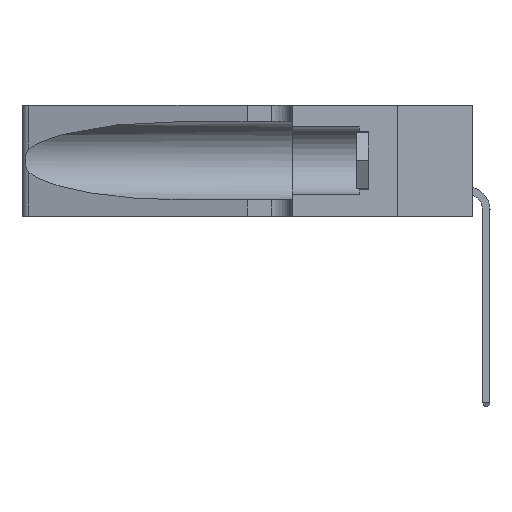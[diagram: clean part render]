
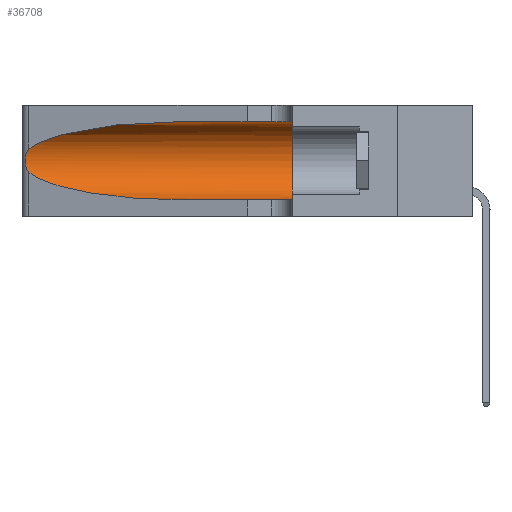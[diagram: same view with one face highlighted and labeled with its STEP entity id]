
A CAD part, left-side view. The second image highlights one B-rep face of the part: STEP entity #36708.
In plain terms, the highlighted cylindrical face has radius 3.308 mm (diameter 6.617 mm), a partial arc.
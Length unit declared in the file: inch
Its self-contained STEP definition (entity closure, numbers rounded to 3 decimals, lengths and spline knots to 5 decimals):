
#712 = CARTESIAN_POINT ( 'NONE',  ( 0.1305, 0.35, 0.185 ) ) ;
#1859 = AXIS2_PLACEMENT_3D ( 'NONE', #20855, #46440, #28651 ) ;
#2155 = EDGE_CURVE ( 'NONE', #11063, #16759, #9258, .T. ) ;
#3030 = DIRECTION ( 'NONE',  ( 0., -1., 0. ) ) ;
#3733 = ORIENTED_EDGE ( 'NONE', *, *, #29926, .T. ) ;
#4401 = CARTESIAN_POINT ( 'NONE',  ( 0.1305, 0.72297, 0.05475 ) ) ;
#5048 = CARTESIAN_POINT ( 'NONE',  ( 0.1305, 0.72297, 0.31525 ) ) ;
#6110 = EDGE_CURVE ( 'NONE', #7838, #38302, #18617, .T. ) ;
#6890 = CARTESIAN_POINT ( 'NONE',  ( 0.25487, 1.22718, 0.14631 ) ) ;
#7838 = VERTEX_POINT ( 'NONE', #35083 ) ;
#9044 = CARTESIAN_POINT ( 'NONE',  ( 0.2373, 1.15595, 0.28018 ) ) ;
#9096 = CARTESIAN_POINT ( 'NONE',  ( 0.25639, 1.23184, 0.21858 ) ) ;
#9258 =( BOUNDED_CURVE ( )  B_SPLINE_CURVE ( 3, ( #15347, #33433, #19290, #4401 ),
 .UNSPECIFIED., .F., .T. ) 
 B_SPLINE_CURVE_WITH_KNOTS ( ( 4, 4 ),
 ( 3.44316, 4.71239 ),
 .UNSPECIFIED. ) 
 CURVE ( )  GEOMETRIC_REPRESENTATION_ITEM ( )  RATIONAL_B_SPLINE_CURVE ( ( 1., 0.87, 0.87, 1. ) ) 
 REPRESENTATION_ITEM ( '' )  );
#9522 = ORIENTED_EDGE ( 'NONE', *, *, #32097, .F. ) ;
#10184 = ORIENTED_EDGE ( 'NONE', *, *, #16195, .T. ) ;
#11063 = VERTEX_POINT ( 'NONE', #45719 ) ;
#11932 = ORIENTED_EDGE ( 'NONE', *, *, #17534, .T. ) ;
#12338 = CARTESIAN_POINT ( 'NONE',  ( 0.25487, 1.22718, 0.22369 ) ) ;
#12715 = CARTESIAN_POINT ( 'NONE',  ( 0.25787, 1.23484, 0.2124 ) ) ;
#15347 = CARTESIAN_POINT ( 'NONE',  ( 0.25487, 1.22718, 0.14631 ) ) ;
#16195 = EDGE_CURVE ( 'NONE', #16759, #22867, #17653, .T. ) ;
#16316 = CARTESIAN_POINT ( 'NONE',  ( 0.1305, 0.35, 0.31525 ) ) ;
#16713 = CARTESIAN_POINT ( 'NONE',  ( 0.26017, 1.23833, 0.17102 ) ) ;
#16759 = VERTEX_POINT ( 'NONE', #20033 ) ;
#16831 = B_SPLINE_CURVE_WITH_KNOTS ( 'NONE', 3,
 ( #30952, #24330, #9096, #12715, #38059, #41662, #34634, #41838, #16713, #42008, #20325, #23975, #42804, #6890 ),
 .UNSPECIFIED., .F., .F.,
 ( 4, 2, 2, 2, 2, 2, 4 ),
 ( 0., 0.00027, 0.00053, 0.00107, 0.0016, 0.00187, 0.00214 ),
 .UNSPECIFIED. ) ;
#17534 = EDGE_CURVE ( 'NONE', #7838, #41190, #37066, .T. ) ;
#17653 = LINE ( 'NONE', #33801, #40776 ) ;
#18617 = LINE ( 'NONE', #31819, #38499 ) ;
#19290 = CARTESIAN_POINT ( 'NONE',  ( 0.18966, 0.96281, 0.05475 ) ) ;
#20033 = CARTESIAN_POINT ( 'NONE',  ( 0.1305, 0.72297, 0.05475 ) ) ;
#20325 = CARTESIAN_POINT ( 'NONE',  ( 0.25789, 1.23486, 0.15765 ) ) ;
#20855 = CARTESIAN_POINT ( 'NONE',  ( 0.1305, 1.61858, 0.185 ) ) ;
#22108 = CARTESIAN_POINT ( 'NONE',  ( 0.25487, 1.22718, 0.22369 ) ) ;
#22867 = VERTEX_POINT ( 'NONE', #43048 ) ;
#23152 = DIRECTION ( 'NONE',  ( 0., -1., 0. ) ) ;
#23975 = CARTESIAN_POINT ( 'NONE',  ( 0.25639, 1.23186, 0.15144 ) ) ;
#24330 = CARTESIAN_POINT ( 'NONE',  ( 0.25555, 1.22994, 0.2215 ) ) ;
#26096 = DIRECTION ( 'NONE',  ( 0., 0., 1. ) ) ;
#26104 = FACE_OUTER_BOUND ( 'NONE', #38270, .T. ) ;
#26655 = ORIENTED_EDGE ( 'NONE', *, *, #2155, .T. ) ;
#26684 = CYLINDRICAL_SURFACE ( 'NONE', #1859, 0.13025 ) ;
#27728 = CIRCLE ( 'NONE', #39976, 0.13025 ) ;
#28651 = DIRECTION ( 'NONE',  ( 0., 0., -1. ) ) ;
#29926 = EDGE_CURVE ( 'NONE', #41190, #11063, #16831, .T. ) ;
#30432 = ORIENTED_EDGE ( 'NONE', *, *, #6110, .F. ) ;
#30952 = CARTESIAN_POINT ( 'NONE',  ( 0.25487, 1.22718, 0.22369 ) ) ;
#31819 = CARTESIAN_POINT ( 'NONE',  ( 0.1305, 1.61858, 0.31525 ) ) ;
#32097 = EDGE_CURVE ( 'NONE', #38302, #22867, #27728, .T. ) ;
#33433 = CARTESIAN_POINT ( 'NONE',  ( 0.2373, 1.15595, 0.08982 ) ) ;
#33801 = CARTESIAN_POINT ( 'NONE',  ( 0.1305, 1.61858, 0.05475 ) ) ;
#34634 = CARTESIAN_POINT ( 'NONE',  ( 0.26075, 1.23896, 0.19203 ) ) ;
#35083 = CARTESIAN_POINT ( 'NONE',  ( 0.1305, 0.72297, 0.31525 ) ) ;
#36708 = ADVANCED_FACE ( 'NONE', ( #26104 ), #26684, .F. ) ;
#37066 =( BOUNDED_CURVE ( )  B_SPLINE_CURVE ( 3, ( #5048, #37850, #9044, #12338 ),
 .UNSPECIFIED., .F., .F. ) 
 B_SPLINE_CURVE_WITH_KNOTS ( ( 4, 4 ),
 ( 1.5708, 2.84003 ),
 .UNSPECIFIED. ) 
 CURVE ( )  GEOMETRIC_REPRESENTATION_ITEM ( )  RATIONAL_B_SPLINE_CURVE ( ( 1., 0.87, 0.87, 1. ) ) 
 REPRESENTATION_ITEM ( '' )  );
#37850 = CARTESIAN_POINT ( 'NONE',  ( 0.18966, 0.96281, 0.31525 ) ) ;
#38059 = CARTESIAN_POINT ( 'NONE',  ( 0.25854, 1.2359, 0.20912 ) ) ;
#38270 = EDGE_LOOP ( 'NONE', ( #11932, #3733, #26655, #10184, #9522, #30432 ) ) ;
#38302 = VERTEX_POINT ( 'NONE', #16316 ) ;
#38499 = VECTOR ( 'NONE', #3030, 39.37008 ) ;
#39976 = AXIS2_PLACEMENT_3D ( 'NONE', #712, #40508, #26096 ) ;
#40508 = DIRECTION ( 'NONE',  ( 0., 1., 0. ) ) ;
#40776 = VECTOR ( 'NONE', #23152, 39.37008 ) ;
#41190 = VERTEX_POINT ( 'NONE', #22108 ) ;
#41662 = CARTESIAN_POINT ( 'NONE',  ( 0.26018, 1.23835, 0.19895 ) ) ;
#41838 = CARTESIAN_POINT ( 'NONE',  ( 0.26075, 1.23896, 0.178 ) ) ;
#42008 = CARTESIAN_POINT ( 'NONE',  ( 0.25856, 1.23593, 0.16098 ) ) ;
#42804 = CARTESIAN_POINT ( 'NONE',  ( 0.25555, 1.22993, 0.14849 ) ) ;
#43048 = CARTESIAN_POINT ( 'NONE',  ( 0.1305, 0.35, 0.05475 ) ) ;
#45719 = CARTESIAN_POINT ( 'NONE',  ( 0.25487, 1.22718, 0.14631 ) ) ;
#46440 = DIRECTION ( 'NONE',  ( 0., -1., 0. ) ) ;
